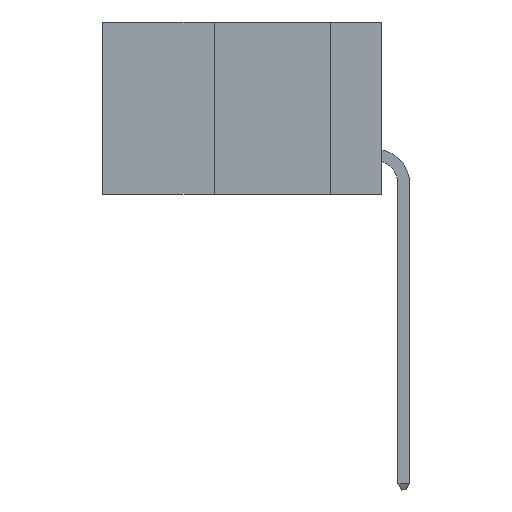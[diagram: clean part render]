
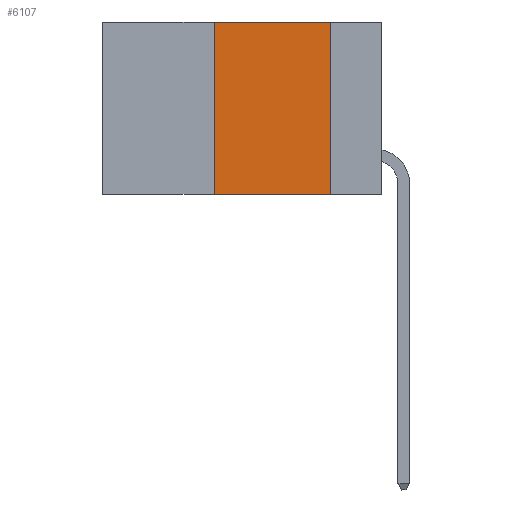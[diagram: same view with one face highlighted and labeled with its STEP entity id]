
A CAD part, left-side view. The second image highlights one B-rep face of the part: STEP entity #6107.
In plain terms, the highlighted planar face has unit normal (-1, 0, 0).
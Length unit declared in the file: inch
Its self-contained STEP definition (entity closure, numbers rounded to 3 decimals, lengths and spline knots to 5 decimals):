
#283 = EDGE_CURVE ( 'NONE', #16213, #17410, #14656, .T. ) ;
#716 = CARTESIAN_POINT ( 'NONE',  ( 0., 0.11, -0.37 ) ) ;
#874 = DIRECTION ( 'NONE',  ( 0., 0., -1. ) ) ;
#1629 = ORIENTED_EDGE ( 'NONE', *, *, #283, .F. ) ;
#1751 = VERTEX_POINT ( 'NONE', #10939 ) ;
#2748 = PLANE ( 'NONE',  #16397 ) ;
#2823 = EDGE_CURVE ( 'NONE', #1751, #16213, #12730, .T. ) ;
#3082 = CARTESIAN_POINT ( 'NONE',  ( 0., 0.6, 0. ) ) ;
#4214 = CARTESIAN_POINT ( 'NONE',  ( 0., 0.6, 0. ) ) ;
#4577 = VECTOR ( 'NONE', #23327, 39.37008 ) ;
#5775 = CARTESIAN_POINT ( 'NONE',  ( 0., 0.36, 0. ) ) ;
#5954 = ORIENTED_EDGE ( 'NONE', *, *, #22565, .F. ) ;
#6081 = EDGE_CURVE ( 'NONE', #1751, #16472, #8625, .T. ) ;
#6107 = ADVANCED_FACE ( 'NONE', ( #23092 ), #2748, .F. ) ;
#6159 = CARTESIAN_POINT ( 'NONE',  ( 0., 0.36, 0. ) ) ;
#8625 = LINE ( 'NONE', #14340, #24026 ) ;
#8855 = DIRECTION ( 'NONE',  ( 0., 0., -1. ) ) ;
#10043 = DIRECTION ( 'NONE',  ( 0., -1., 0. ) ) ;
#10583 = EDGE_LOOP ( 'NONE', ( #5954, #1629, #16386, #15388 ) ) ;
#10791 = DIRECTION ( 'NONE',  ( 0., -1., 0. ) ) ;
#10939 = CARTESIAN_POINT ( 'NONE',  ( 0., 0.36, -0.37 ) ) ;
#11017 = VECTOR ( 'NONE', #10043, 39.37008 ) ;
#12727 = CARTESIAN_POINT ( 'NONE',  ( 0., 0.11, 0. ) ) ;
#12730 = LINE ( 'NONE', #5775, #4577 ) ;
#14340 = CARTESIAN_POINT ( 'NONE',  ( 0., 0.6, -0.37 ) ) ;
#14656 = LINE ( 'NONE', #4214, #11017 ) ;
#15388 = ORIENTED_EDGE ( 'NONE', *, *, #6081, .T. ) ;
#15489 = CARTESIAN_POINT ( 'NONE',  ( 0., 0.11, 0. ) ) ;
#16013 = VECTOR ( 'NONE', #8855, 39.37008 ) ;
#16213 = VERTEX_POINT ( 'NONE', #6159 ) ;
#16334 = LINE ( 'NONE', #12727, #16013 ) ;
#16386 = ORIENTED_EDGE ( 'NONE', *, *, #2823, .F. ) ;
#16397 = AXIS2_PLACEMENT_3D ( 'NONE', #3082, #23940, #874 ) ;
#16472 = VERTEX_POINT ( 'NONE', #716 ) ;
#17410 = VERTEX_POINT ( 'NONE', #15489 ) ;
#22565 = EDGE_CURVE ( 'NONE', #17410, #16472, #16334, .T. ) ;
#23092 = FACE_OUTER_BOUND ( 'NONE', #10583, .T. ) ;
#23327 = DIRECTION ( 'NONE',  ( 0., 0., 1. ) ) ;
#23940 = DIRECTION ( 'NONE',  ( 1., 0., 0. ) ) ;
#24026 = VECTOR ( 'NONE', #10791, 39.37008 ) ;
